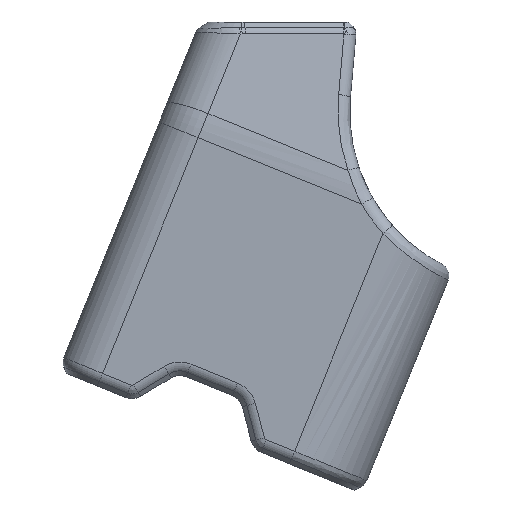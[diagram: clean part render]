
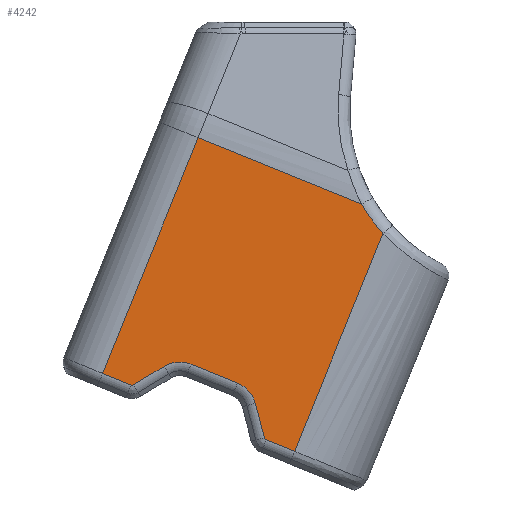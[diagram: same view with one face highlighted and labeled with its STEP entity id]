
A CAD part, left-side view. The second image highlights one B-rep face of the part: STEP entity #4242.
In plain terms, the highlighted planar face has unit normal (-1, 0, 0).
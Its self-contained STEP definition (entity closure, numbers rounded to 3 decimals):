
#349=PLANE('',#4662);
#521=FACE_OUTER_BOUND('',#800,.T.);
#800=EDGE_LOOP('',(#3333,#3334,#3335,#3336,#3337,#3338,#3339,#3340,#3341,
#3342,#3343,#3344,#3345));
#1094=LINE('',#7080,#1370);
#1095=LINE('',#7096,#1371);
#1096=LINE('',#7104,#1372);
#1097=LINE('',#7112,#1373);
#1098=LINE('',#7128,#1374);
#1110=LINE('',#7369,#1386);
#1111=LINE('',#7373,#1387);
#1112=LINE('',#7374,#1388);
#1370=VECTOR('',#5414,10.);
#1371=VECTOR('',#5423,10.);
#1372=VECTOR('',#5434,10.);
#1373=VECTOR('',#5445,10.);
#1374=VECTOR('',#5454,10.);
#1386=VECTOR('',#5566,10.);
#1387=VECTOR('',#5569,10.);
#1388=VECTOR('',#5570,10.);
#1586=CIRCLE('',#4596,0.379);
#1589=CIRCLE('',#4601,3.621);
#1592=CIRCLE('',#4606,3.621);
#1595=CIRCLE('',#4610,0.379);
#1629=CIRCLE('',#4663,22.);
#1857=VERTEX_POINT('',#7076);
#1858=VERTEX_POINT('',#7078);
#1859=VERTEX_POINT('',#7090);
#1860=VERTEX_POINT('',#7094);
#1861=VERTEX_POINT('',#7098);
#1862=VERTEX_POINT('',#7102);
#1863=VERTEX_POINT('',#7106);
#1864=VERTEX_POINT('',#7110);
#1865=VERTEX_POINT('',#7122);
#1866=VERTEX_POINT('',#7126);
#1889=VERTEX_POINT('',#7368);
#1890=VERTEX_POINT('',#7370);
#1891=VERTEX_POINT('',#7372);
#2347=EDGE_CURVE('',#1858,#1857,#1094,.T.);
#2349=EDGE_CURVE('',#1859,#1858,#1586,.T.);
#2351=EDGE_CURVE('',#1860,#1859,#1095,.T.);
#2353=EDGE_CURVE('',#1861,#1860,#1589,.T.);
#2355=EDGE_CURVE('',#1862,#1861,#1096,.T.);
#2357=EDGE_CURVE('',#1863,#1862,#1592,.T.);
#2359=EDGE_CURVE('',#1864,#1863,#1097,.T.);
#2361=EDGE_CURVE('',#1865,#1864,#1595,.T.);
#2363=EDGE_CURVE('',#1866,#1865,#1098,.T.);
#2409=EDGE_CURVE('',#1866,#1889,#1110,.T.);
#2410=EDGE_CURVE('',#1890,#1889,#1629,.T.);
#2411=EDGE_CURVE('',#1891,#1890,#1111,.T.);
#2412=EDGE_CURVE('',#1857,#1891,#1112,.T.);
#3333=ORIENTED_EDGE('',*,*,#2409,.T.);
#3334=ORIENTED_EDGE('',*,*,#2410,.F.);
#3335=ORIENTED_EDGE('',*,*,#2411,.F.);
#3336=ORIENTED_EDGE('',*,*,#2412,.F.);
#3337=ORIENTED_EDGE('',*,*,#2347,.F.);
#3338=ORIENTED_EDGE('',*,*,#2349,.F.);
#3339=ORIENTED_EDGE('',*,*,#2351,.F.);
#3340=ORIENTED_EDGE('',*,*,#2353,.F.);
#3341=ORIENTED_EDGE('',*,*,#2355,.F.);
#3342=ORIENTED_EDGE('',*,*,#2357,.F.);
#3343=ORIENTED_EDGE('',*,*,#2359,.F.);
#3344=ORIENTED_EDGE('',*,*,#2361,.F.);
#3345=ORIENTED_EDGE('',*,*,#2363,.F.);
#4242=ADVANCED_FACE('',(#521),#349,.F.);
#4596=AXIS2_PLACEMENT_3D('',#7092,#5417,#5418);
#4601=AXIS2_PLACEMENT_3D('',#7100,#5428,#5429);
#4606=AXIS2_PLACEMENT_3D('',#7108,#5439,#5440);
#4610=AXIS2_PLACEMENT_3D('',#7124,#5448,#5449);
#4662=AXIS2_PLACEMENT_3D('',#7367,#5564,#5565);
#4663=AXIS2_PLACEMENT_3D('',#7371,#5567,#5568);
#5414=DIRECTION('',(0.,0.927,0.376));
#5417=DIRECTION('center_axis',(1.,0.,0.));
#5418=DIRECTION('ref_axis',(0.,-0.079,-0.997));
#5423=DIRECTION('',(0.,0.856,-0.517));
#5428=DIRECTION('center_axis',(-1.,0.,0.));
#5429=DIRECTION('ref_axis',(0.,0.079,0.997));
#5434=DIRECTION('',(0.,0.927,0.376));
#5439=DIRECTION('center_axis',(-1.,0.,0.));
#5440=DIRECTION('ref_axis',(0.,-0.751,0.66));
#5445=DIRECTION('',(0.,0.254,0.967));
#5448=DIRECTION('center_axis',(1.,0.,0.));
#5449=DIRECTION('ref_axis',(0.,0.751,-0.66));
#5454=DIRECTION('',(0.,0.927,0.376));
#5564=DIRECTION('center_axis',(1.,0.,0.));
#5565=DIRECTION('ref_axis',(0.,0.927,0.376));
#5566=DIRECTION('',(0.,-0.376,0.927));
#5567=DIRECTION('center_axis',(-1.,0.,0.));
#5568=DIRECTION('ref_axis',(0.,0.794,-0.608));
#5569=DIRECTION('',(0.,-0.927,-0.376));
#5570=DIRECTION('',(0.,-0.376,0.927));
#7076=CARTESIAN_POINT('',(-14.419,1.113,78.017));
#7078=CARTESIAN_POINT('',(-14.419,-2.286,76.639));
#7080=CARTESIAN_POINT('',(-14.419,-19.509,69.655));
#7090=CARTESIAN_POINT('',(-14.419,-2.625,76.666));
#7092=CARTESIAN_POINT('Origin',(-14.419,-2.429,76.99));
#7094=CARTESIAN_POINT('',(-14.419,-6.25,78.858));
#7096=CARTESIAN_POINT('',(-14.419,-10.84,81.633));
#7098=CARTESIAN_POINT('',(-14.419,-9.485,79.115));
#7100=CARTESIAN_POINT('Origin',(-14.419,-8.124,75.759));
#7102=CARTESIAN_POINT('',(-14.419,-15.041,76.862));
#7104=CARTESIAN_POINT('',(-14.419,-21.812,74.116));
#7106=CARTESIAN_POINT('',(-14.419,-17.183,74.425));
#7108=CARTESIAN_POINT('Origin',(-14.419,-13.68,73.506));
#7110=CARTESIAN_POINT('',(-14.419,-18.258,70.326));
#7112=CARTESIAN_POINT('',(-14.419,-19.044,67.329));
#7122=CARTESIAN_POINT('',(-14.419,-18.482,70.071));
#7124=CARTESIAN_POINT('Origin',(-14.419,-18.624,70.422));
#7126=CARTESIAN_POINT('',(-14.419,-21.881,68.693));
#7128=CARTESIAN_POINT('',(-14.419,-19.509,69.655));
#7367=CARTESIAN_POINT('Origin',(-14.419,-19.393,62.557));
#7368=CARTESIAN_POINT('',(-14.419,-32.451,94.759));
#7369=CARTESIAN_POINT('',(-14.419,-19.393,62.557));
#7370=CARTESIAN_POINT('',(-14.419,-29.92,98.294));
#7371=CARTESIAN_POINT('Origin',(-14.419,-48.984,109.273));
#7372=CARTESIAN_POINT('',(-14.419,-10.331,106.237));
#7373=CARTESIAN_POINT('',(-14.419,-22.031,101.493));
#7374=CARTESIAN_POINT('',(-14.419,1.722,76.515));
